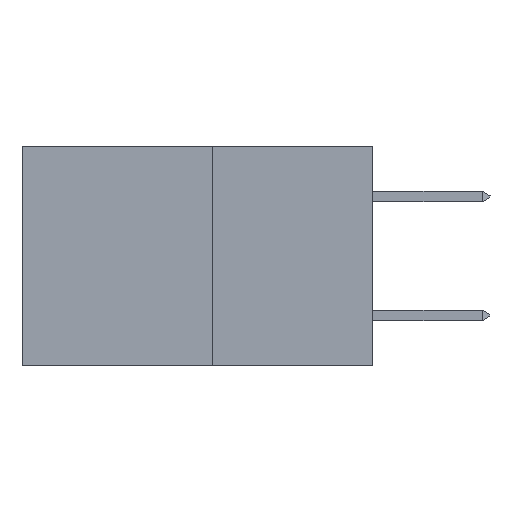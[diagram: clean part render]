
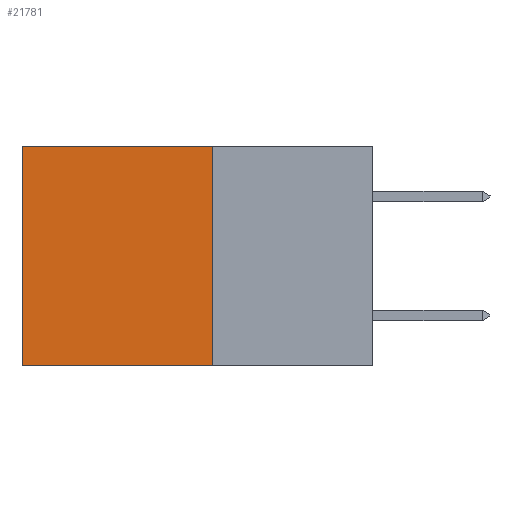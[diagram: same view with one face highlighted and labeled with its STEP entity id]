
A CAD part, left-side view. The second image highlights one B-rep face of the part: STEP entity #21781.
In plain terms, the highlighted planar face has unit normal (-1, 0, 0).
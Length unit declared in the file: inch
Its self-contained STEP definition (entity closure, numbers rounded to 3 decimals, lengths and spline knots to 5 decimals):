
#385 = CARTESIAN_POINT ( 'NONE',  ( 0.277, 0.59, -0.37 ) ) ;
#589 = ORIENTED_EDGE ( 'NONE', *, *, #9691, .T. ) ;
#1102 = VECTOR ( 'NONE', #2450, 39.37008 ) ;
#2450 = DIRECTION ( 'NONE',  ( 0., 1., 0. ) ) ;
#2681 = ORIENTED_EDGE ( 'NONE', *, *, #7204, .F. ) ;
#4734 = CARTESIAN_POINT ( 'NONE',  ( 0.277, 0.59, 0. ) ) ;
#7204 = EDGE_CURVE ( 'NONE', #21048, #18915, #14251, .T. ) ;
#7697 = AXIS2_PLACEMENT_3D ( 'NONE', #10009, #27864, #14541 ) ;
#7835 = CARTESIAN_POINT ( 'NONE',  ( 0.277, 0.27, 0. ) ) ;
#9477 = CARTESIAN_POINT ( 'NONE',  ( 0.277, 0.27, -0.37 ) ) ;
#9691 = EDGE_CURVE ( 'NONE', #17415, #24265, #26991, .T. ) ;
#10009 = CARTESIAN_POINT ( 'NONE',  ( 0.277, 0.27, -0.37 ) ) ;
#10430 = LINE ( 'NONE', #25956, #21692 ) ;
#11344 = EDGE_LOOP ( 'NONE', ( #589, #20236, #2681, #27976 ) ) ;
#11699 = FACE_OUTER_BOUND ( 'NONE', #11344, .T. ) ;
#14251 = LINE ( 'NONE', #9477, #25407 ) ;
#14541 = DIRECTION ( 'NONE',  ( 0., 0., -1. ) ) ;
#14869 = DIRECTION ( 'NONE',  ( 0., 1., 0. ) ) ;
#17415 = VERTEX_POINT ( 'NONE', #4734 ) ;
#18116 = EDGE_CURVE ( 'NONE', #18915, #24265, #19285, .T. ) ;
#18915 = VERTEX_POINT ( 'NONE', #22927 ) ;
#19143 = EDGE_CURVE ( 'NONE', #21048, #17415, #10430, .T. ) ;
#19285 = LINE ( 'NONE', #22794, #1102 ) ;
#20236 = ORIENTED_EDGE ( 'NONE', *, *, #18116, .F. ) ;
#20439 = VECTOR ( 'NONE', #22968, 39.37008 ) ;
#21048 = VERTEX_POINT ( 'NONE', #7835 ) ;
#21692 = VECTOR ( 'NONE', #14869, 39.37008 ) ;
#21781 = ADVANCED_FACE ( 'NONE', ( #11699 ), #25628, .F. ) ;
#22794 = CARTESIAN_POINT ( 'NONE',  ( 0.277, 0.27, -0.37 ) ) ;
#22927 = CARTESIAN_POINT ( 'NONE',  ( 0.277, 0.27, -0.37 ) ) ;
#22968 = DIRECTION ( 'NONE',  ( 0., 0., -1. ) ) ;
#24265 = VERTEX_POINT ( 'NONE', #385 ) ;
#24662 = DIRECTION ( 'NONE',  ( 0., 0., -1. ) ) ;
#25147 = CARTESIAN_POINT ( 'NONE',  ( 0.277, 0.59, -0.37 ) ) ;
#25407 = VECTOR ( 'NONE', #24662, 39.37008 ) ;
#25628 = PLANE ( 'NONE',  #7697 ) ;
#25956 = CARTESIAN_POINT ( 'NONE',  ( 0.277, 0.27, 0. ) ) ;
#26991 = LINE ( 'NONE', #25147, #20439 ) ;
#27864 = DIRECTION ( 'NONE',  ( 1., 0., 0. ) ) ;
#27976 = ORIENTED_EDGE ( 'NONE', *, *, #19143, .T. ) ;
